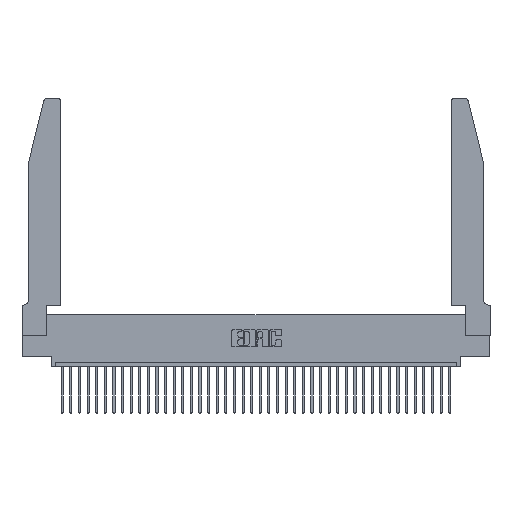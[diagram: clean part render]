
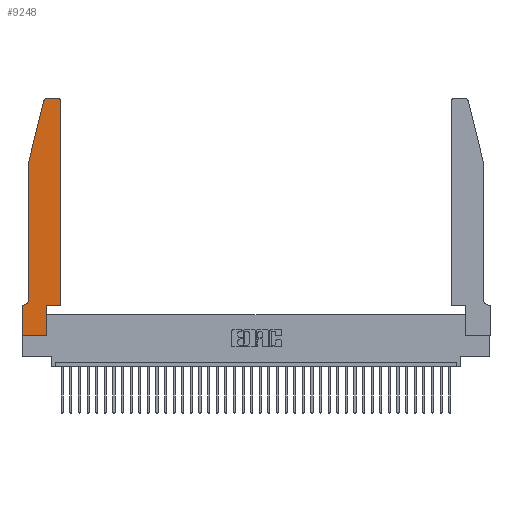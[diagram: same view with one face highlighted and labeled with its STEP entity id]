
A CAD part, top view. The second image highlights one B-rep face of the part: STEP entity #9248.
In plain terms, the highlighted planar face has unit normal (0, 0, 1).
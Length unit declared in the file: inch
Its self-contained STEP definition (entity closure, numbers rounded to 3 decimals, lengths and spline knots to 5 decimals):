
#852 = CARTESIAN_POINT ( 'NONE',  ( 0.2865, 0., 0.37 ) ) ;
#1030 = LINE ( 'NONE', #37770, #32180 ) ;
#1373 = DIRECTION ( 'NONE',  ( 0., 0., 1. ) ) ;
#1784 = CARTESIAN_POINT ( 'NONE',  ( 0.2605, 2.75, 0.37 ) ) ;
#2180 = CARTESIAN_POINT ( 'NONE',  ( 0., 0., 0.37 ) ) ;
#2658 = CARTESIAN_POINT ( 'NONE',  ( 0.284, 2.72, 0.37 ) ) ;
#2991 = CARTESIAN_POINT ( 'NONE',  ( 0.0755, 2., 0.37 ) ) ;
#4033 = DIRECTION ( 'NONE',  ( 1., 0., 0. ) ) ;
#4749 = DIRECTION ( 'NONE',  ( -0.239, -0.971, 0. ) ) ;
#4913 = CARTESIAN_POINT ( 'NONE',  ( 0.4505, 2.72, 0.37 ) ) ;
#5510 = LINE ( 'NONE', #30558, #11589 ) ;
#5652 = DIRECTION ( 'NONE',  ( -1., 0., 0. ) ) ;
#6474 = CARTESIAN_POINT ( 'NONE',  ( 0., 0., 0.37 ) ) ;
#6587 = DIRECTION ( 'NONE',  ( 1., 0., 0. ) ) ;
#6753 = CARTESIAN_POINT ( 'NONE',  ( 0., 0.35, 0.37 ) ) ;
#6821 = AXIS2_PLACEMENT_3D ( 'NONE', #30987, #1373, #34032 ) ;
#7558 = VECTOR ( 'NONE', #38613, 39.37008 ) ;
#8246 = LINE ( 'NONE', #31396, #38392 ) ;
#8300 = AXIS2_PLACEMENT_3D ( 'NONE', #2658, #35334, #23753 ) ;
#8546 = DIRECTION ( 'NONE',  ( 0., 0., -1. ) ) ;
#8785 = ORIENTED_EDGE ( 'NONE', *, *, #36744, .T. ) ;
#9248 = ADVANCED_FACE ( 'NONE', ( #36904 ), #15928, .T. ) ;
#9644 = ORIENTED_EDGE ( 'NONE', *, *, #24650, .T. ) ;
#9898 = ORIENTED_EDGE ( 'NONE', *, *, #18015, .T. ) ;
#10066 = VERTEX_POINT ( 'NONE', #23465 ) ;
#10461 = CARTESIAN_POINT ( 'NONE',  ( 0.0055, 0.35, 0.37 ) ) ;
#10489 = EDGE_CURVE ( 'NONE', #15530, #19510, #1030, .T. ) ;
#10498 = CIRCLE ( 'NONE', #8300, 0.03 ) ;
#11395 = LINE ( 'NONE', #37205, #20409 ) ;
#11417 = CARTESIAN_POINT ( 'NONE',  ( 0.4205, 2.72, 0.37 ) ) ;
#11589 = VECTOR ( 'NONE', #6587, 39.37008 ) ;
#11672 = CIRCLE ( 'NONE', #13782, 0.07 ) ;
#12470 = LINE ( 'NONE', #1784, #25740 ) ;
#12912 = DIRECTION ( 'NONE',  ( 0., -1., 0. ) ) ;
#13782 = AXIS2_PLACEMENT_3D ( 'NONE', #35563, #8546, #5652 ) ;
#13791 = ORIENTED_EDGE ( 'NONE', *, *, #35084, .T. ) ;
#14725 = DIRECTION ( 'NONE',  ( 0., 0., 1. ) ) ;
#15402 = ORIENTED_EDGE ( 'NONE', *, *, #25089, .T. ) ;
#15530 = VERTEX_POINT ( 'NONE', #16921 ) ;
#15917 = VECTOR ( 'NONE', #12912, 39.37008 ) ;
#15928 = PLANE ( 'NONE',  #6821 ) ;
#15987 = LINE ( 'NONE', #22114, #16976 ) ;
#16258 = EDGE_CURVE ( 'NONE', #32320, #23202, #15987, .T. ) ;
#16479 = LINE ( 'NONE', #32735, #7558 ) ;
#16921 = CARTESIAN_POINT ( 'NONE',  ( 0.25487, 2.72718, 0.37 ) ) ;
#16976 = VECTOR ( 'NONE', #30918, 39.37008 ) ;
#18015 = EDGE_CURVE ( 'NONE', #23202, #21783, #24024, .T. ) ;
#18478 = CIRCLE ( 'NONE', #33507, 0.03 ) ;
#19510 = VERTEX_POINT ( 'NONE', #2991 ) ;
#19734 = ORIENTED_EDGE ( 'NONE', *, *, #16258, .T. ) ;
#20288 = CARTESIAN_POINT ( 'NONE',  ( 0.284, 2.75, 0.37 ) ) ;
#20409 = VECTOR ( 'NONE', #25512, 39.37008 ) ;
#20850 = CARTESIAN_POINT ( 'NONE',  ( 0.2865, 0.35, 0.37 ) ) ;
#21783 = VERTEX_POINT ( 'NONE', #2180 ) ;
#22004 = DIRECTION ( 'NONE',  ( 0., 1., 0. ) ) ;
#22114 = CARTESIAN_POINT ( 'NONE',  ( 0.0755, 0.35, 0.37 ) ) ;
#22308 = ORIENTED_EDGE ( 'NONE', *, *, #22833, .T. ) ;
#22833 = EDGE_CURVE ( 'NONE', #19510, #10066, #11395, .T. ) ;
#23202 = VERTEX_POINT ( 'NONE', #6753 ) ;
#23465 = CARTESIAN_POINT ( 'NONE',  ( 0.0755, 0.42, 0.37 ) ) ;
#23673 = EDGE_CURVE ( 'NONE', #35383, #28082, #16479, .T. ) ;
#23753 = DIRECTION ( 'NONE',  ( 1., 0., 0. ) ) ;
#23794 = CARTESIAN_POINT ( 'NONE',  ( 0.4505, 0.35, 0.37 ) ) ;
#23895 = EDGE_LOOP ( 'NONE', ( #9644, #26051, #35074, #22308, #13791, #19734, #9898, #24463, #36388, #15402, #34780, #8785 ) ) ;
#24024 = LINE ( 'NONE', #6474, #15917 ) ;
#24301 = VERTEX_POINT ( 'NONE', #27767 ) ;
#24463 = ORIENTED_EDGE ( 'NONE', *, *, #35870, .T. ) ;
#24650 = EDGE_CURVE ( 'NONE', #24301, #38872, #12470, .T. ) ;
#25089 = EDGE_CURVE ( 'NONE', #28082, #30675, #8246, .T. ) ;
#25512 = DIRECTION ( 'NONE',  ( 0., -1., 0. ) ) ;
#25740 = VECTOR ( 'NONE', #38091, 39.37008 ) ;
#26051 = ORIENTED_EDGE ( 'NONE', *, *, #32013, .T. ) ;
#26602 = VERTEX_POINT ( 'NONE', #4913 ) ;
#27085 = EDGE_CURVE ( 'NONE', #30675, #26602, #31545, .T. ) ;
#27767 = CARTESIAN_POINT ( 'NONE',  ( 0.4205, 2.75, 0.37 ) ) ;
#28082 = VERTEX_POINT ( 'NONE', #20850 ) ;
#30558 = CARTESIAN_POINT ( 'NONE',  ( 0., 0., 0.37 ) ) ;
#30675 = VERTEX_POINT ( 'NONE', #23794 ) ;
#30918 = DIRECTION ( 'NONE',  ( -1., 0., 0. ) ) ;
#30949 = CARTESIAN_POINT ( 'NONE',  ( 0.4505, 0.35, 0.37 ) ) ;
#30987 = CARTESIAN_POINT ( 'NONE',  ( 0., 0.35, 0.37 ) ) ;
#31396 = CARTESIAN_POINT ( 'NONE',  ( 0.4505, 0.35, 0.37 ) ) ;
#31545 = LINE ( 'NONE', #30949, #34374 ) ;
#32013 = EDGE_CURVE ( 'NONE', #38872, #15530, #10498, .T. ) ;
#32180 = VECTOR ( 'NONE', #4749, 39.37008 ) ;
#32320 = VERTEX_POINT ( 'NONE', #10461 ) ;
#32735 = CARTESIAN_POINT ( 'NONE',  ( 0.2865, 0.35, 0.37 ) ) ;
#33507 = AXIS2_PLACEMENT_3D ( 'NONE', #11417, #14725, #35317 ) ;
#34032 = DIRECTION ( 'NONE',  ( 1., 0., 0. ) ) ;
#34374 = VECTOR ( 'NONE', #22004, 39.37008 ) ;
#34780 = ORIENTED_EDGE ( 'NONE', *, *, #27085, .T. ) ;
#35074 = ORIENTED_EDGE ( 'NONE', *, *, #10489, .T. ) ;
#35084 = EDGE_CURVE ( 'NONE', #10066, #32320, #11672, .T. ) ;
#35317 = DIRECTION ( 'NONE',  ( 1., 0., 0. ) ) ;
#35334 = DIRECTION ( 'NONE',  ( 0., 0., 1. ) ) ;
#35383 = VERTEX_POINT ( 'NONE', #852 ) ;
#35563 = CARTESIAN_POINT ( 'NONE',  ( 0.0055, 0.42, 0.37 ) ) ;
#35870 = EDGE_CURVE ( 'NONE', #21783, #35383, #5510, .T. ) ;
#36388 = ORIENTED_EDGE ( 'NONE', *, *, #23673, .T. ) ;
#36744 = EDGE_CURVE ( 'NONE', #26602, #24301, #18478, .T. ) ;
#36904 = FACE_OUTER_BOUND ( 'NONE', #23895, .T. ) ;
#37205 = CARTESIAN_POINT ( 'NONE',  ( 0.0755, 2., 0.37 ) ) ;
#37770 = CARTESIAN_POINT ( 'NONE',  ( 0.0755, 2., 0.37 ) ) ;
#38091 = DIRECTION ( 'NONE',  ( -1., 0., 0. ) ) ;
#38392 = VECTOR ( 'NONE', #4033, 39.37008 ) ;
#38613 = DIRECTION ( 'NONE',  ( 0., 1., 0. ) ) ;
#38872 = VERTEX_POINT ( 'NONE', #20288 ) ;
